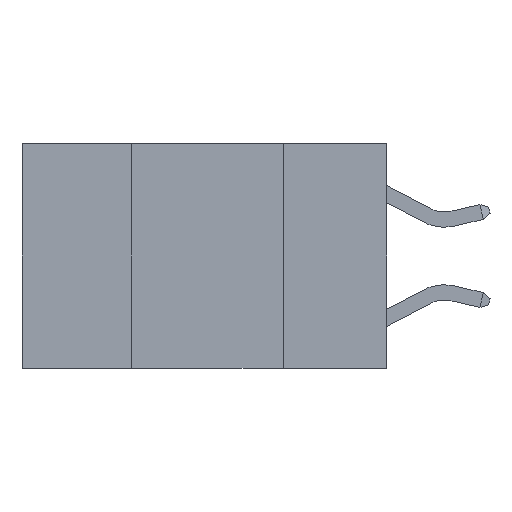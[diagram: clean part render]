
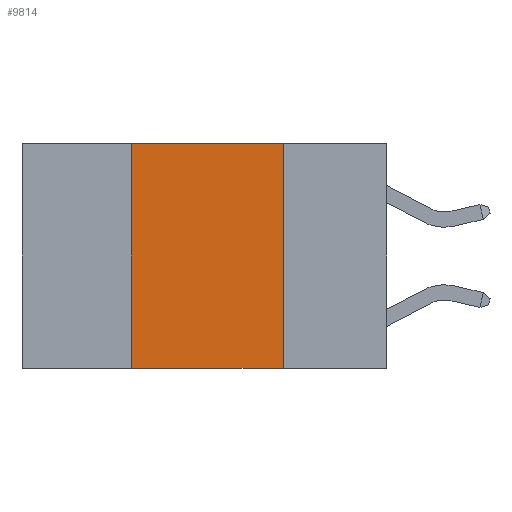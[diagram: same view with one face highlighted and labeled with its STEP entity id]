
A CAD part, left-side view. The second image highlights one B-rep face of the part: STEP entity #9814.
In plain terms, the highlighted planar face has unit normal (-1, 0, 0).
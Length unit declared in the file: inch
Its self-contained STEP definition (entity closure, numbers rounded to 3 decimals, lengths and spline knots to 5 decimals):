
#424 = DIRECTION ( 'NONE',  ( 0., -1., 0. ) ) ;
#915 = EDGE_CURVE ( 'NONE', #15183, #3287, #15503, .T. ) ;
#1178 = EDGE_CURVE ( 'NONE', #3287, #6913, #2186, .T. ) ;
#1205 = EDGE_CURVE ( 'NONE', #9810, #15183, #10261, .T. ) ;
#2003 = CARTESIAN_POINT ( 'NONE',  ( 0., 0.42, -0.37 ) ) ;
#2186 = LINE ( 'NONE', #16687, #13656 ) ;
#2402 = DIRECTION ( 'NONE',  ( 0., -1., 0. ) ) ;
#3239 = CARTESIAN_POINT ( 'NONE',  ( 0., 0.6, 0. ) ) ;
#3287 = VERTEX_POINT ( 'NONE', #5671 ) ;
#3694 = EDGE_CURVE ( 'NONE', #9810, #6913, #9723, .T. ) ;
#4605 = ORIENTED_EDGE ( 'NONE', *, *, #915, .F. ) ;
#4726 = EDGE_LOOP ( 'NONE', ( #16808, #4605, #5602, #11790 ) ) ;
#4785 = AXIS2_PLACEMENT_3D ( 'NONE', #3239, #13779, #15296 ) ;
#5602 = ORIENTED_EDGE ( 'NONE', *, *, #1205, .F. ) ;
#5604 = CARTESIAN_POINT ( 'NONE',  ( 0., 0.42, 0. ) ) ;
#5671 = CARTESIAN_POINT ( 'NONE',  ( 0., 0.17, 0. ) ) ;
#6030 = VECTOR ( 'NONE', #424, 39.37008 ) ;
#6913 = VERTEX_POINT ( 'NONE', #9144 ) ;
#7501 = DIRECTION ( 'NONE',  ( 0., 0., -1. ) ) ;
#8144 = VECTOR ( 'NONE', #2402, 39.37008 ) ;
#9144 = CARTESIAN_POINT ( 'NONE',  ( 0., 0.17, -0.37 ) ) ;
#9723 = LINE ( 'NONE', #13831, #6030 ) ;
#9810 = VERTEX_POINT ( 'NONE', #2003 ) ;
#9814 = ADVANCED_FACE ( 'NONE', ( #11112 ), #12575, .F. ) ;
#10261 = LINE ( 'NONE', #12916, #13944 ) ;
#11112 = FACE_OUTER_BOUND ( 'NONE', #4726, .T. ) ;
#11704 = DIRECTION ( 'NONE',  ( 0., 0., 1. ) ) ;
#11790 = ORIENTED_EDGE ( 'NONE', *, *, #3694, .T. ) ;
#12575 = PLANE ( 'NONE',  #4785 ) ;
#12916 = CARTESIAN_POINT ( 'NONE',  ( 0., 0.42, 0. ) ) ;
#13656 = VECTOR ( 'NONE', #7501, 39.37008 ) ;
#13779 = DIRECTION ( 'NONE',  ( 1., 0., 0. ) ) ;
#13831 = CARTESIAN_POINT ( 'NONE',  ( 0., 0.6, -0.37 ) ) ;
#13944 = VECTOR ( 'NONE', #11704, 39.37008 ) ;
#14236 = CARTESIAN_POINT ( 'NONE',  ( 0., 0.6, 0. ) ) ;
#15183 = VERTEX_POINT ( 'NONE', #5604 ) ;
#15296 = DIRECTION ( 'NONE',  ( 0., 0., -1. ) ) ;
#15503 = LINE ( 'NONE', #14236, #8144 ) ;
#16687 = CARTESIAN_POINT ( 'NONE',  ( 0., 0.17, 0. ) ) ;
#16808 = ORIENTED_EDGE ( 'NONE', *, *, #1178, .F. ) ;
